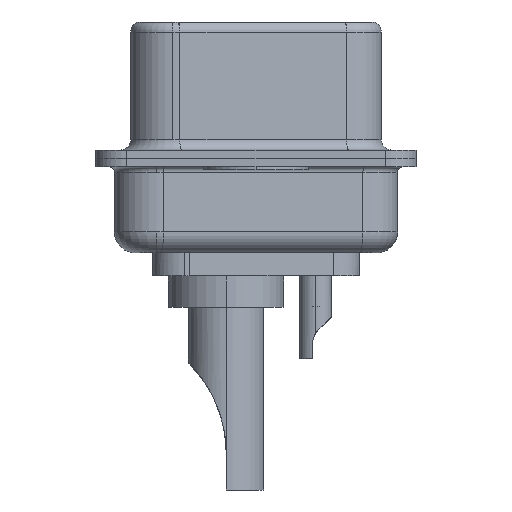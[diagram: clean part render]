
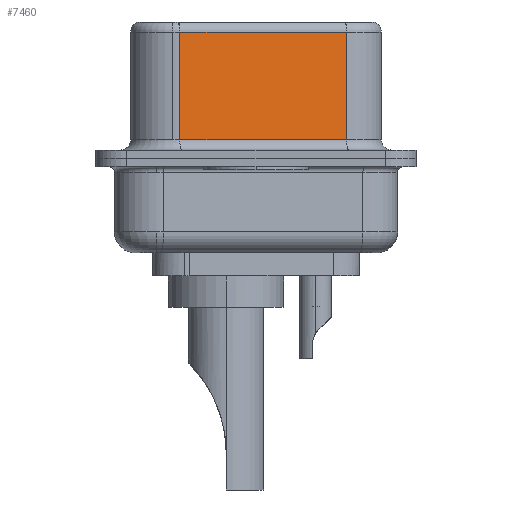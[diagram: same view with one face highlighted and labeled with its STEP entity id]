
A CAD part, left-side view. The second image highlights one B-rep face of the part: STEP entity #7460.
In plain terms, the highlighted planar face has unit normal (-0.985, -0.174, 0).
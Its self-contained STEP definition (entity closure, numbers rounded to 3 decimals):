
#626 = DIRECTION ( 'NONE',  ( -0.174, 0.985, 0. ) ) ;
#1955 = CARTESIAN_POINT ( 'NONE',  ( 3.73, 3.628, 6.02 ) ) ;
#3608 = CARTESIAN_POINT ( 'NONE',  ( 5.132, -4.322, 6.52 ) ) ;
#3735 = DIRECTION ( 'NONE',  ( 0.174, -0.985, 0. ) ) ;
#4570 = LINE ( 'NONE', #17282, #8656 ) ;
#5166 = CARTESIAN_POINT ( 'NONE',  ( 3.73, 3.628, 0.9 ) ) ;
#5793 = VERTEX_POINT ( 'NONE', #1955 ) ;
#6326 = CARTESIAN_POINT ( 'NONE',  ( 5.132, -4.322, 6.02 ) ) ;
#6626 = VECTOR ( 'NONE', #7662, 1000. ) ;
#6782 = AXIS2_PLACEMENT_3D ( 'NONE', #3608, #9750, #626 ) ;
#6996 = EDGE_CURVE ( 'NONE', #13134, #5793, #18702, .T. ) ;
#7150 = CARTESIAN_POINT ( 'NONE',  ( 3.73, 3.628, 6.52 ) ) ;
#7460 = ADVANCED_FACE ( 'NONE', ( #8052 ), #8158, .F. ) ;
#7508 = EDGE_CURVE ( 'NONE', #9667, #10237, #19427, .T. ) ;
#7662 = DIRECTION ( 'NONE',  ( -0.174, 0.985, 0. ) ) ;
#8052 = FACE_OUTER_BOUND ( 'NONE', #14674, .T. ) ;
#8158 = PLANE ( 'NONE',  #6782 ) ;
#8656 = VECTOR ( 'NONE', #15758, 1000. ) ;
#9667 = VERTEX_POINT ( 'NONE', #5166 ) ;
#9750 = DIRECTION ( 'NONE',  ( 0.985, 0.174, 0. ) ) ;
#9876 = VECTOR ( 'NONE', #16229, 1000. ) ;
#10237 = VERTEX_POINT ( 'NONE', #14363 ) ;
#10370 = EDGE_CURVE ( 'NONE', #5793, #9667, #13392, .T. ) ;
#10950 = VECTOR ( 'NONE', #3735, 1000. ) ;
#11334 = CARTESIAN_POINT ( 'NONE',  ( 5.132, -4.322, 0.9 ) ) ;
#13069 = ORIENTED_EDGE ( 'NONE', *, *, #16130, .F. ) ;
#13134 = VERTEX_POINT ( 'NONE', #6326 ) ;
#13392 = LINE ( 'NONE', #7150, #9876 ) ;
#14363 = CARTESIAN_POINT ( 'NONE',  ( 5.132, -4.322, 0.9 ) ) ;
#14674 = EDGE_LOOP ( 'NONE', ( #13069, #15241, #16573, #15234 ) ) ;
#15194 = CARTESIAN_POINT ( 'NONE',  ( 5.132, -4.322, 6.02 ) ) ;
#15234 = ORIENTED_EDGE ( 'NONE', *, *, #7508, .T. ) ;
#15241 = ORIENTED_EDGE ( 'NONE', *, *, #6996, .T. ) ;
#15758 = DIRECTION ( 'NONE',  ( 0., 0., -1. ) ) ;
#16130 = EDGE_CURVE ( 'NONE', #13134, #10237, #4570, .T. ) ;
#16229 = DIRECTION ( 'NONE',  ( 0., 0., -1. ) ) ;
#16573 = ORIENTED_EDGE ( 'NONE', *, *, #10370, .T. ) ;
#17282 = CARTESIAN_POINT ( 'NONE',  ( 5.132, -4.322, 6.52 ) ) ;
#18702 = LINE ( 'NONE', #15194, #6626 ) ;
#19427 = LINE ( 'NONE', #11334, #10950 ) ;
